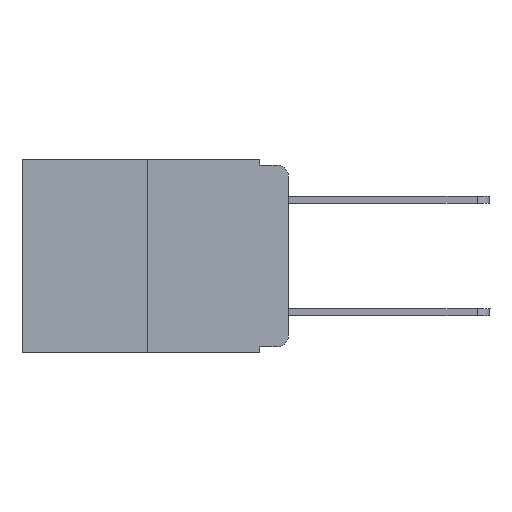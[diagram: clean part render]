
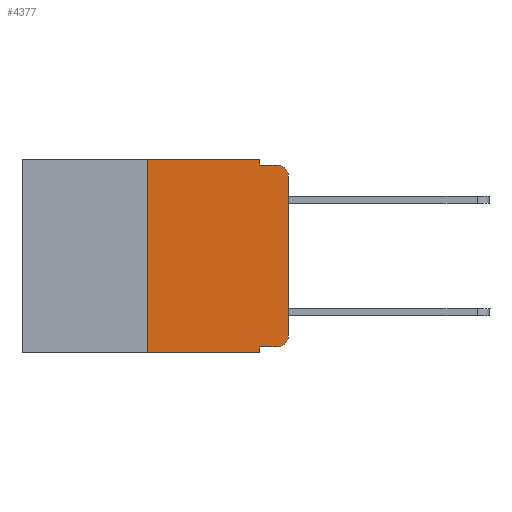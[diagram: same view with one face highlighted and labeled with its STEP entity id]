
A CAD part, left-side view. The second image highlights one B-rep face of the part: STEP entity #4377.
In plain terms, the highlighted planar face has unit normal (-1, 0, 0).
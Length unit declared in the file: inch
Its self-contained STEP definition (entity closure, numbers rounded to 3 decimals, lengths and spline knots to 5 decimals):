
#104 = DIRECTION ( 'NONE',  ( 0., 0., 1. ) ) ;
#169 = CARTESIAN_POINT ( 'NONE',  ( 0., 0.051, -0.01 ) ) ;
#173 = EDGE_LOOP ( 'NONE', ( #4639, #2900, #10847, #5118, #5465, #10233, #12606, #9149, #9372, #3435 ) ) ;
#545 = VECTOR ( 'NONE', #14270, 39.37008 ) ;
#713 = DIRECTION ( 'NONE',  ( 0., -1., 0. ) ) ;
#1029 = CARTESIAN_POINT ( 'NONE',  ( 0., 0.051, -0.01 ) ) ;
#1108 = DIRECTION ( 'NONE',  ( 0., -1., 0. ) ) ;
#1232 = EDGE_CURVE ( 'NONE', #12110, #3375, #9300, .T. ) ;
#1290 = LINE ( 'NONE', #10781, #4348 ) ;
#1677 = VERTEX_POINT ( 'NONE', #11292 ) ;
#1725 = CARTESIAN_POINT ( 'NONE',  ( 0., 0., -0.03 ) ) ;
#1839 = DIRECTION ( 'NONE',  ( -1., 0., 0. ) ) ;
#1891 = CARTESIAN_POINT ( 'NONE',  ( 0., 0.02, -0.313 ) ) ;
#2154 = CARTESIAN_POINT ( 'NONE',  ( 0., 0.051, 0. ) ) ;
#2276 = PLANE ( 'NONE',  #15003 ) ;
#2283 = AXIS2_PLACEMENT_3D ( 'NONE', #10249, #1839, #12688 ) ;
#2482 = CARTESIAN_POINT ( 'NONE',  ( 0., 0.25, 0. ) ) ;
#2900 = ORIENTED_EDGE ( 'NONE', *, *, #5130, .T. ) ;
#3074 = AXIS2_PLACEMENT_3D ( 'NONE', #1891, #3297, #10294 ) ;
#3297 = DIRECTION ( 'NONE',  ( -1., 0., 0. ) ) ;
#3327 = VECTOR ( 'NONE', #12854, 39.37008 ) ;
#3375 = VERTEX_POINT ( 'NONE', #10992 ) ;
#3435 = ORIENTED_EDGE ( 'NONE', *, *, #10827, .T. ) ;
#4051 = LINE ( 'NONE', #12550, #5757 ) ;
#4165 = CARTESIAN_POINT ( 'NONE',  ( 0., 0.473, -0.343 ) ) ;
#4234 = VERTEX_POINT ( 'NONE', #1725 ) ;
#4348 = VECTOR ( 'NONE', #104, 39.37008 ) ;
#4377 = ADVANCED_FACE ( 'NONE', ( #8474 ), #2276, .F. ) ;
#4606 = CARTESIAN_POINT ( 'NONE',  ( 0., 0.051, -0.333 ) ) ;
#4639 = ORIENTED_EDGE ( 'NONE', *, *, #12501, .T. ) ;
#4644 = EDGE_CURVE ( 'NONE', #3375, #14851, #4051, .T. ) ;
#5118 = ORIENTED_EDGE ( 'NONE', *, *, #4644, .F. ) ;
#5130 = EDGE_CURVE ( 'NONE', #4234, #13970, #8038, .T. ) ;
#5308 = DIRECTION ( 'NONE',  ( 0., 0., -1. ) ) ;
#5465 = ORIENTED_EDGE ( 'NONE', *, *, #1232, .F. ) ;
#5757 = VECTOR ( 'NONE', #5308, 39.37008 ) ;
#5899 = CARTESIAN_POINT ( 'NONE',  ( 0., 0.02, -0.01 ) ) ;
#6001 = EDGE_CURVE ( 'NONE', #14851, #13970, #9338, .T. ) ;
#6097 = CARTESIAN_POINT ( 'NONE',  ( 0., 0.051, -0.333 ) ) ;
#6373 = CARTESIAN_POINT ( 'NONE',  ( 0., 0.051, -0.343 ) ) ;
#6674 = LINE ( 'NONE', #4165, #6899 ) ;
#6899 = VECTOR ( 'NONE', #713, 39.37008 ) ;
#7019 = DIRECTION ( 'NONE',  ( 0., 0., -1. ) ) ;
#7099 = CARTESIAN_POINT ( 'NONE',  ( 0., 0.25, -0.343 ) ) ;
#7283 = EDGE_CURVE ( 'NONE', #15526, #14544, #6674, .T. ) ;
#7377 = CARTESIAN_POINT ( 'NONE',  ( 0., 0.473, 0. ) ) ;
#7442 = CARTESIAN_POINT ( 'NONE',  ( 0., 0.02, -0.333 ) ) ;
#8038 = CIRCLE ( 'NONE', #2283, 0.02 ) ;
#8052 = VERTEX_POINT ( 'NONE', #7442 ) ;
#8474 = FACE_OUTER_BOUND ( 'NONE', #173, .T. ) ;
#8547 = DIRECTION ( 'NONE',  ( 1., 0., 0. ) ) ;
#8666 = EDGE_CURVE ( 'NONE', #15526, #12110, #12581, .T. ) ;
#8738 = VECTOR ( 'NONE', #11563, 39.37008 ) ;
#8970 = CARTESIAN_POINT ( 'NONE',  ( 0., 0.25, 0. ) ) ;
#9149 = ORIENTED_EDGE ( 'NONE', *, *, #14207, .F. ) ;
#9300 = LINE ( 'NONE', #15374, #3327 ) ;
#9338 = LINE ( 'NONE', #1029, #12948 ) ;
#9372 = ORIENTED_EDGE ( 'NONE', *, *, #11815, .T. ) ;
#10233 = ORIENTED_EDGE ( 'NONE', *, *, #8666, .F. ) ;
#10249 = CARTESIAN_POINT ( 'NONE',  ( 0., 0.02, -0.03 ) ) ;
#10294 = DIRECTION ( 'NONE',  ( 0., 0., -1. ) ) ;
#10552 = LINE ( 'NONE', #2154, #15198 ) ;
#10730 = LINE ( 'NONE', #4606, #545 ) ;
#10781 = CARTESIAN_POINT ( 'NONE',  ( 0., 0., 0. ) ) ;
#10827 = EDGE_CURVE ( 'NONE', #8052, #1677, #14843, .T. ) ;
#10847 = ORIENTED_EDGE ( 'NONE', *, *, #6001, .F. ) ;
#10992 = CARTESIAN_POINT ( 'NONE',  ( 0., 0.051, 0. ) ) ;
#11292 = CARTESIAN_POINT ( 'NONE',  ( 0., 0., -0.313 ) ) ;
#11534 = VERTEX_POINT ( 'NONE', #6097 ) ;
#11563 = DIRECTION ( 'NONE',  ( 0., 0., 1. ) ) ;
#11815 = EDGE_CURVE ( 'NONE', #11534, #8052, #10730, .T. ) ;
#12110 = VERTEX_POINT ( 'NONE', #2482 ) ;
#12174 = DIRECTION ( 'NONE',  ( 0., 0., -1. ) ) ;
#12501 = EDGE_CURVE ( 'NONE', #1677, #4234, #1290, .T. ) ;
#12550 = CARTESIAN_POINT ( 'NONE',  ( 0., 0.051, 0. ) ) ;
#12581 = LINE ( 'NONE', #8970, #8738 ) ;
#12606 = ORIENTED_EDGE ( 'NONE', *, *, #7283, .T. ) ;
#12688 = DIRECTION ( 'NONE',  ( 0., 0., -1. ) ) ;
#12854 = DIRECTION ( 'NONE',  ( 0., -1., 0. ) ) ;
#12948 = VECTOR ( 'NONE', #1108, 39.37008 ) ;
#13970 = VERTEX_POINT ( 'NONE', #5899 ) ;
#14207 = EDGE_CURVE ( 'NONE', #11534, #14544, #10552, .T. ) ;
#14270 = DIRECTION ( 'NONE',  ( 0., -1., 0. ) ) ;
#14544 = VERTEX_POINT ( 'NONE', #6373 ) ;
#14843 = CIRCLE ( 'NONE', #3074, 0.02 ) ;
#14851 = VERTEX_POINT ( 'NONE', #169 ) ;
#15003 = AXIS2_PLACEMENT_3D ( 'NONE', #7377, #8547, #12174 ) ;
#15198 = VECTOR ( 'NONE', #7019, 39.37008 ) ;
#15374 = CARTESIAN_POINT ( 'NONE',  ( 0., 0.473, 0. ) ) ;
#15526 = VERTEX_POINT ( 'NONE', #7099 ) ;
